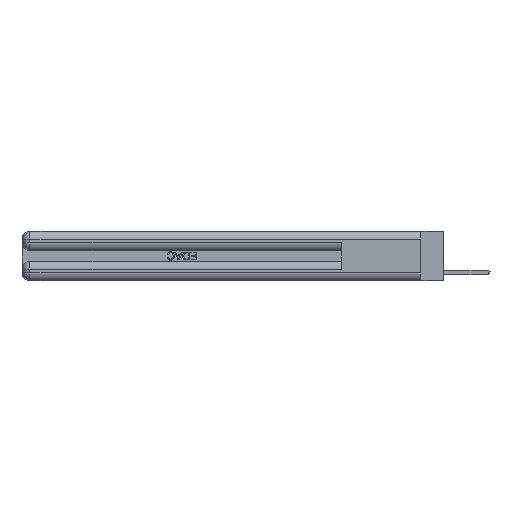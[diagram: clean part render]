
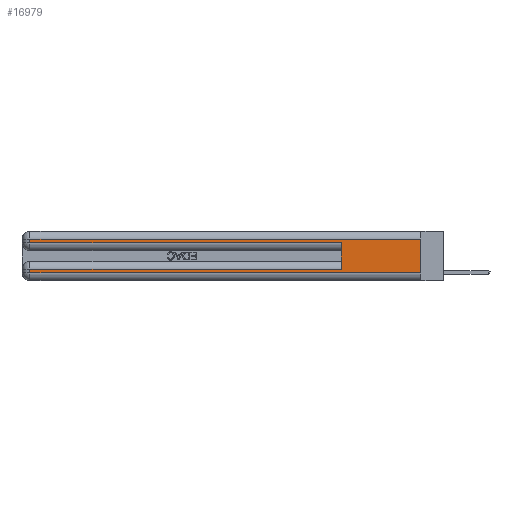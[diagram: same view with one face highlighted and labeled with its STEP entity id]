
A CAD part, left-side view. The second image highlights one B-rep face of the part: STEP entity #16979.
In plain terms, the highlighted planar face has unit normal (-1, 0, 0).
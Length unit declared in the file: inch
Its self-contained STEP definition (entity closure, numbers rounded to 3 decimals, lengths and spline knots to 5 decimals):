
#507 = ORIENTED_EDGE ( 'NONE', *, *, #15127, .T. ) ;
#538 = LINE ( 'NONE', #25802, #11577 ) ;
#712 = CARTESIAN_POINT ( 'NONE',  ( 0., 0., 0.37 ) ) ;
#813 = CARTESIAN_POINT ( 'NONE',  ( 0., 0., 0.06 ) ) ;
#1085 = CARTESIAN_POINT ( 'NONE',  ( 0., 2.94, 0.085 ) ) ;
#1601 = CARTESIAN_POINT ( 'NONE',  ( 0., 0., 0.31 ) ) ;
#1689 = EDGE_CURVE ( 'NONE', #24798, #16239, #28999, .T. ) ;
#1980 = CARTESIAN_POINT ( 'NONE',  ( 0., 0., 0.06 ) ) ;
#2224 = CARTESIAN_POINT ( 'NONE',  ( 0., 0.6, 0.285 ) ) ;
#2489 = CARTESIAN_POINT ( 'NONE',  ( 0., 2.94, 0.37 ) ) ;
#2509 = ORIENTED_EDGE ( 'NONE', *, *, #14669, .T. ) ;
#2596 = ORIENTED_EDGE ( 'NONE', *, *, #6976, .F. ) ;
#3031 = EDGE_LOOP ( 'NONE', ( #11260, #20711, #507, #19549, #2596, #22972, #2509, #19979 ) ) ;
#3374 = DIRECTION ( 'NONE',  ( 0., -1., 0. ) ) ;
#3858 = CARTESIAN_POINT ( 'NONE',  ( 0., 0.6, 0.145 ) ) ;
#4149 = VECTOR ( 'NONE', #16248, 39.37008 ) ;
#4648 = EDGE_CURVE ( 'NONE', #16562, #18156, #538, .T. ) ;
#5935 = VECTOR ( 'NONE', #7957, 39.37008 ) ;
#6976 = EDGE_CURVE ( 'NONE', #24798, #18156, #26911, .T. ) ;
#7005 = LINE ( 'NONE', #22091, #5935 ) ;
#7957 = DIRECTION ( 'NONE',  ( 0., 0., -1. ) ) ;
#8679 = CARTESIAN_POINT ( 'NONE',  ( 0., 0.6, 0.085 ) ) ;
#10316 = VECTOR ( 'NONE', #3374, 39.37008 ) ;
#10468 = DIRECTION ( 'NONE',  ( 0., 1., 0. ) ) ;
#10670 = LINE ( 'NONE', #813, #10316 ) ;
#10958 = FACE_OUTER_BOUND ( 'NONE', #3031, .T. ) ;
#11260 = ORIENTED_EDGE ( 'NONE', *, *, #14445, .F. ) ;
#11577 = VECTOR ( 'NONE', #23608, 39.37008 ) ;
#11949 = VERTEX_POINT ( 'NONE', #27700 ) ;
#12270 = CARTESIAN_POINT ( 'NONE',  ( 0., 2.94, 0.06 ) ) ;
#12335 = VERTEX_POINT ( 'NONE', #21885 ) ;
#12433 = VERTEX_POINT ( 'NONE', #1980 ) ;
#12451 = DIRECTION ( 'NONE',  ( 1., 0., 0. ) ) ;
#12524 = VECTOR ( 'NONE', #10468, 39.37008 ) ;
#12936 = VECTOR ( 'NONE', #27162, 39.37008 ) ;
#14445 = EDGE_CURVE ( 'NONE', #12335, #12433, #7005, .T. ) ;
#14591 = CARTESIAN_POINT ( 'NONE',  ( 0., 2.94, 0.37 ) ) ;
#14669 = EDGE_CURVE ( 'NONE', #16239, #15335, #18028, .T. ) ;
#15127 = EDGE_CURVE ( 'NONE', #11949, #16562, #17263, .T. ) ;
#15335 = VERTEX_POINT ( 'NONE', #12270 ) ;
#16239 = VERTEX_POINT ( 'NONE', #1085 ) ;
#16248 = DIRECTION ( 'NONE',  ( 0., 0., 1. ) ) ;
#16562 = VERTEX_POINT ( 'NONE', #17597 ) ;
#16979 = ADVANCED_FACE ( 'NONE', ( #10958 ), #26768, .F. ) ;
#17263 = LINE ( 'NONE', #2489, #19813 ) ;
#17597 = CARTESIAN_POINT ( 'NONE',  ( 0., 2.94, 0.285 ) ) ;
#18028 = LINE ( 'NONE', #14591, #22781 ) ;
#18156 = VERTEX_POINT ( 'NONE', #2224 ) ;
#19549 = ORIENTED_EDGE ( 'NONE', *, *, #4648, .T. ) ;
#19788 = CARTESIAN_POINT ( 'NONE',  ( 0., 0., 0.085 ) ) ;
#19813 = VECTOR ( 'NONE', #30045, 39.37008 ) ;
#19979 = ORIENTED_EDGE ( 'NONE', *, *, #24776, .T. ) ;
#20711 = ORIENTED_EDGE ( 'NONE', *, *, #26760, .T. ) ;
#21885 = CARTESIAN_POINT ( 'NONE',  ( 0., 0., 0.31 ) ) ;
#21933 = DIRECTION ( 'NONE',  ( 0., 0., -1. ) ) ;
#22091 = CARTESIAN_POINT ( 'NONE',  ( 0., 0., 0.37 ) ) ;
#22781 = VECTOR ( 'NONE', #26256, 39.37008 ) ;
#22972 = ORIENTED_EDGE ( 'NONE', *, *, #1689, .T. ) ;
#23608 = DIRECTION ( 'NONE',  ( 0., -1., 0. ) ) ;
#24776 = EDGE_CURVE ( 'NONE', #15335, #12433, #10670, .T. ) ;
#24798 = VERTEX_POINT ( 'NONE', #8679 ) ;
#24833 = AXIS2_PLACEMENT_3D ( 'NONE', #712, #12451, #21933 ) ;
#25802 = CARTESIAN_POINT ( 'NONE',  ( 0., 0., 0.285 ) ) ;
#26256 = DIRECTION ( 'NONE',  ( 0., 0., -1. ) ) ;
#26760 = EDGE_CURVE ( 'NONE', #12335, #11949, #29079, .T. ) ;
#26768 = PLANE ( 'NONE',  #24833 ) ;
#26911 = LINE ( 'NONE', #3858, #4149 ) ;
#27162 = DIRECTION ( 'NONE',  ( 0., 1., 0. ) ) ;
#27700 = CARTESIAN_POINT ( 'NONE',  ( 0., 2.94, 0.31 ) ) ;
#28999 = LINE ( 'NONE', #19788, #12524 ) ;
#29079 = LINE ( 'NONE', #1601, #12936 ) ;
#30045 = DIRECTION ( 'NONE',  ( 0., 0., -1. ) ) ;
